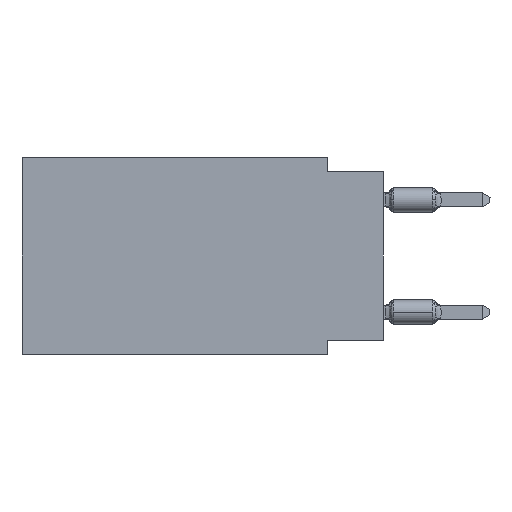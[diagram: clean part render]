
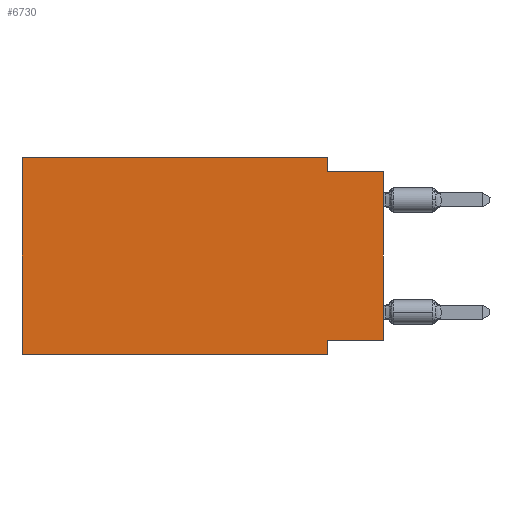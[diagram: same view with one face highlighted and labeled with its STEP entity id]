
A CAD part, left-side view. The second image highlights one B-rep face of the part: STEP entity #6730.
In plain terms, the highlighted planar face has unit normal (-1, 0, 0).
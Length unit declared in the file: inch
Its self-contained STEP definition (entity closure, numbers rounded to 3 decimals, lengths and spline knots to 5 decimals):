
#1659 = ORIENTED_EDGE ( 'NONE', *, *, #15501, .F. ) ;
#1784 = CARTESIAN_POINT ( 'NONE',  ( 0., 0., -0.025 ) ) ;
#4550 = FACE_OUTER_BOUND ( 'NONE', #32392, .T. ) ;
#4652 = VECTOR ( 'NONE', #32841, 39.37008 ) ;
#5030 = LINE ( 'NONE', #22222, #42512 ) ;
#5728 = ORIENTED_EDGE ( 'NONE', *, *, #18564, .F. ) ;
#6175 = VERTEX_POINT ( 'NONE', #14683 ) ;
#6380 = CARTESIAN_POINT ( 'NONE',  ( 0., 0.1, 0. ) ) ;
#6730 = ADVANCED_FACE ( 'NONE', ( #4550 ), #27583, .F. ) ;
#7870 = CARTESIAN_POINT ( 'NONE',  ( 0., 0., 0. ) ) ;
#8043 = EDGE_CURVE ( 'NONE', #8835, #11378, #8129, .T. ) ;
#8129 = LINE ( 'NONE', #14805, #4652 ) ;
#8684 = CARTESIAN_POINT ( 'NONE',  ( 0., 0.1, 0. ) ) ;
#8835 = VERTEX_POINT ( 'NONE', #35837 ) ;
#8967 = LINE ( 'NONE', #15393, #31316 ) ;
#9456 = ORIENTED_EDGE ( 'NONE', *, *, #31630, .F. ) ;
#9805 = ORIENTED_EDGE ( 'NONE', *, *, #8043, .T. ) ;
#10953 = ORIENTED_EDGE ( 'NONE', *, *, #11562, .F. ) ;
#11378 = VERTEX_POINT ( 'NONE', #31874 ) ;
#11562 = EDGE_CURVE ( 'NONE', #39362, #29540, #8967, .T. ) ;
#13072 = VECTOR ( 'NONE', #31680, 39.37008 ) ;
#14060 = CARTESIAN_POINT ( 'NONE',  ( 0., 0.645, 0. ) ) ;
#14683 = CARTESIAN_POINT ( 'NONE',  ( 0., 0.645, 0. ) ) ;
#14805 = CARTESIAN_POINT ( 'NONE',  ( 0., 0.645, -0.35 ) ) ;
#14979 = ORIENTED_EDGE ( 'NONE', *, *, #35483, .T. ) ;
#15198 = LINE ( 'NONE', #7870, #45235 ) ;
#15393 = CARTESIAN_POINT ( 'NONE',  ( 0., 0., -0.325 ) ) ;
#15501 = EDGE_CURVE ( 'NONE', #22099, #43454, #37762, .T. ) ;
#16632 = EDGE_CURVE ( 'NONE', #43454, #24063, #5030, .T. ) ;
#17087 = LINE ( 'NONE', #20722, #35261 ) ;
#17095 = CARTESIAN_POINT ( 'NONE',  ( 0., 0.645, 0. ) ) ;
#18175 = DIRECTION ( 'NONE',  ( 0., 0., 1. ) ) ;
#18564 = EDGE_CURVE ( 'NONE', #6175, #22099, #35558, .T. ) ;
#20722 = CARTESIAN_POINT ( 'NONE',  ( 0., 0.1, -0.35 ) ) ;
#21865 = CARTESIAN_POINT ( 'NONE',  ( 0., 0., -0.325 ) ) ;
#22099 = VERTEX_POINT ( 'NONE', #8684 ) ;
#22222 = CARTESIAN_POINT ( 'NONE',  ( 0., 0., -0.025 ) ) ;
#22444 = VECTOR ( 'NONE', #30310, 39.37008 ) ;
#22937 = DIRECTION ( 'NONE',  ( 0., 1., 0. ) ) ;
#24063 = VERTEX_POINT ( 'NONE', #1784 ) ;
#25182 = ORIENTED_EDGE ( 'NONE', *, *, #44086, .F. ) ;
#25772 = AXIS2_PLACEMENT_3D ( 'NONE', #17095, #37683, #34692 ) ;
#27583 = PLANE ( 'NONE',  #25772 ) ;
#27883 = ORIENTED_EDGE ( 'NONE', *, *, #16632, .F. ) ;
#29540 = VERTEX_POINT ( 'NONE', #34234 ) ;
#30310 = DIRECTION ( 'NONE',  ( 0., 0., 1. ) ) ;
#31026 = DIRECTION ( 'NONE',  ( 0., 0., -1. ) ) ;
#31316 = VECTOR ( 'NONE', #22937, 39.37008 ) ;
#31630 = EDGE_CURVE ( 'NONE', #8835, #6175, #34171, .T. ) ;
#31680 = DIRECTION ( 'NONE',  ( 0., -1., 0. ) ) ;
#31874 = CARTESIAN_POINT ( 'NONE',  ( 0., 0.1, -0.35 ) ) ;
#32392 = EDGE_LOOP ( 'NONE', ( #14979, #27883, #1659, #5728, #9456, #9805, #25182, #10953 ) ) ;
#32841 = DIRECTION ( 'NONE',  ( 0., -1., 0. ) ) ;
#34103 = DIRECTION ( 'NONE',  ( 0., 0., -1. ) ) ;
#34171 = LINE ( 'NONE', #41052, #22444 ) ;
#34234 = CARTESIAN_POINT ( 'NONE',  ( 0., 0.1, -0.325 ) ) ;
#34692 = DIRECTION ( 'NONE',  ( 0., 0., -1. ) ) ;
#35261 = VECTOR ( 'NONE', #31026, 39.37008 ) ;
#35483 = EDGE_CURVE ( 'NONE', #39362, #24063, #15198, .T. ) ;
#35558 = LINE ( 'NONE', #14060, #13072 ) ;
#35837 = CARTESIAN_POINT ( 'NONE',  ( 0., 0.645, -0.35 ) ) ;
#36189 = DIRECTION ( 'NONE',  ( 0., -1., 0. ) ) ;
#37683 = DIRECTION ( 'NONE',  ( 1., 0., 0. ) ) ;
#37762 = LINE ( 'NONE', #6380, #43297 ) ;
#39362 = VERTEX_POINT ( 'NONE', #21865 ) ;
#41052 = CARTESIAN_POINT ( 'NONE',  ( 0., 0.645, 0. ) ) ;
#42512 = VECTOR ( 'NONE', #36189, 39.37008 ) ;
#43297 = VECTOR ( 'NONE', #34103, 39.37008 ) ;
#43306 = CARTESIAN_POINT ( 'NONE',  ( 0., 0.1, -0.025 ) ) ;
#43454 = VERTEX_POINT ( 'NONE', #43306 ) ;
#44086 = EDGE_CURVE ( 'NONE', #29540, #11378, #17087, .T. ) ;
#45235 = VECTOR ( 'NONE', #18175, 39.37008 ) ;
